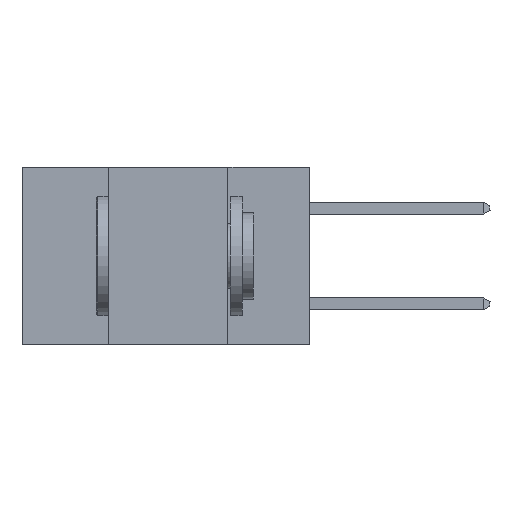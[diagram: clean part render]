
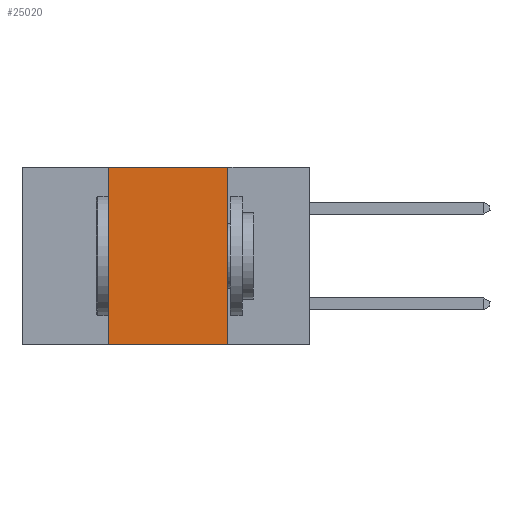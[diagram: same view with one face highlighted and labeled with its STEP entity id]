
A CAD part, left-side view. The second image highlights one B-rep face of the part: STEP entity #25020.
In plain terms, the highlighted planar face has unit normal (-1, 0, 0).
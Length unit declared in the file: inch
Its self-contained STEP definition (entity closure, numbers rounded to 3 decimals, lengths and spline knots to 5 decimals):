
#186 = VECTOR ( 'NONE', #26449, 39.37008 ) ;
#248 = CARTESIAN_POINT ( 'NONE',  ( 0., 0.42, 0. ) ) ;
#3082 = DIRECTION ( 'NONE',  ( 0., 0., -1. ) ) ;
#6562 = LINE ( 'NONE', #32496, #40785 ) ;
#7940 = CARTESIAN_POINT ( 'NONE',  ( 0., 0.17, -0.37 ) ) ;
#8359 = FACE_OUTER_BOUND ( 'NONE', #35267, .T. ) ;
#12489 = VERTEX_POINT ( 'NONE', #19713 ) ;
#13036 = ORIENTED_EDGE ( 'NONE', *, *, #16544, .T. ) ;
#15425 = AXIS2_PLACEMENT_3D ( 'NONE', #40684, #24163, #24881 ) ;
#16226 = ORIENTED_EDGE ( 'NONE', *, *, #37957, .F. ) ;
#16544 = EDGE_CURVE ( 'NONE', #42301, #40076, #35931, .T. ) ;
#17622 = EDGE_CURVE ( 'NONE', #42301, #12489, #41992, .T. ) ;
#18902 = DIRECTION ( 'NONE',  ( 0., -1., 0. ) ) ;
#19713 = CARTESIAN_POINT ( 'NONE',  ( 0., 0.42, 0. ) ) ;
#20494 = EDGE_CURVE ( 'NONE', #42329, #40076, #6562, .T. ) ;
#24163 = DIRECTION ( 'NONE',  ( 1., 0., 0. ) ) ;
#24640 = VECTOR ( 'NONE', #18902, 39.37008 ) ;
#24881 = DIRECTION ( 'NONE',  ( 0., 0., -1. ) ) ;
#25020 = ADVANCED_FACE ( 'NONE', ( #8359 ), #27354, .F. ) ;
#25953 = ORIENTED_EDGE ( 'NONE', *, *, #17622, .F. ) ;
#26299 = CARTESIAN_POINT ( 'NONE',  ( 0., 0.6, -0.37 ) ) ;
#26449 = DIRECTION ( 'NONE',  ( 0., -1., 0. ) ) ;
#27354 = PLANE ( 'NONE',  #15425 ) ;
#28644 = CARTESIAN_POINT ( 'NONE',  ( 0., 0.6, 0. ) ) ;
#32496 = CARTESIAN_POINT ( 'NONE',  ( 0., 0.17, 0. ) ) ;
#32870 = ORIENTED_EDGE ( 'NONE', *, *, #20494, .F. ) ;
#33271 = CARTESIAN_POINT ( 'NONE',  ( 0., 0.42, -0.37 ) ) ;
#33419 = CARTESIAN_POINT ( 'NONE',  ( 0., 0.17, 0. ) ) ;
#33935 = LINE ( 'NONE', #28644, #24640 ) ;
#35267 = EDGE_LOOP ( 'NONE', ( #32870, #16226, #25953, #13036 ) ) ;
#35827 = VECTOR ( 'NONE', #40214, 39.37008 ) ;
#35931 = LINE ( 'NONE', #26299, #186 ) ;
#37957 = EDGE_CURVE ( 'NONE', #12489, #42329, #33935, .T. ) ;
#40076 = VERTEX_POINT ( 'NONE', #7940 ) ;
#40214 = DIRECTION ( 'NONE',  ( 0., 0., 1. ) ) ;
#40684 = CARTESIAN_POINT ( 'NONE',  ( 0., 0.6, 0. ) ) ;
#40785 = VECTOR ( 'NONE', #3082, 39.37008 ) ;
#41992 = LINE ( 'NONE', #248, #35827 ) ;
#42301 = VERTEX_POINT ( 'NONE', #33271 ) ;
#42329 = VERTEX_POINT ( 'NONE', #33419 ) ;
